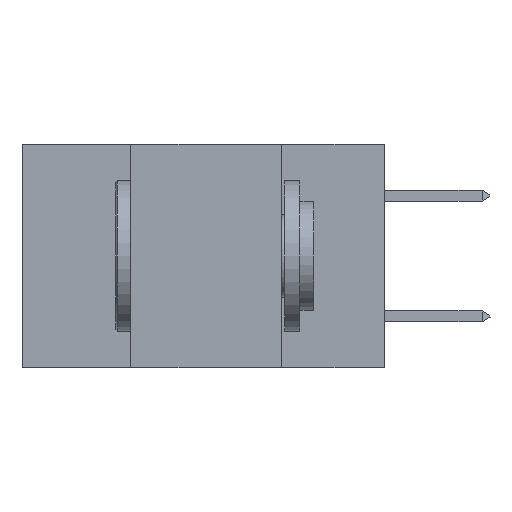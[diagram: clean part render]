
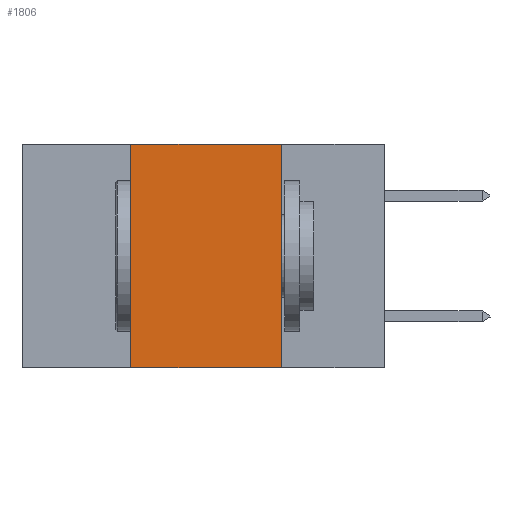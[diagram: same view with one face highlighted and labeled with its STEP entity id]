
A CAD part, left-side view. The second image highlights one B-rep face of the part: STEP entity #1806.
In plain terms, the highlighted planar face has unit normal (-1, 0, 0).
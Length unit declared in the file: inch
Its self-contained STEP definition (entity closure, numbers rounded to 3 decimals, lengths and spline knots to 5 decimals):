
#465 = CARTESIAN_POINT ( 'NONE',  ( 0., 0.42, 0. ) ) ;
#1806 = ADVANCED_FACE ( 'NONE', ( #6356 ), #15922, .F. ) ;
#1963 = ORIENTED_EDGE ( 'NONE', *, *, #30874, .F. ) ;
#4531 = CARTESIAN_POINT ( 'NONE',  ( 0., 0.17, -0.37 ) ) ;
#5035 = VECTOR ( 'NONE', #5827, 39.37008 ) ;
#5827 = DIRECTION ( 'NONE',  ( 0., 0., -1. ) ) ;
#6119 = LINE ( 'NONE', #32080, #33643 ) ;
#6356 = FACE_OUTER_BOUND ( 'NONE', #23006, .T. ) ;
#6683 = CARTESIAN_POINT ( 'NONE',  ( 0., 0.6, -0.37 ) ) ;
#7139 = DIRECTION ( 'NONE',  ( 0., 0., -1. ) ) ;
#7797 = VERTEX_POINT ( 'NONE', #34424 ) ;
#9125 = CARTESIAN_POINT ( 'NONE',  ( 0., 0.17, 0. ) ) ;
#10080 = VECTOR ( 'NONE', #25362, 39.37008 ) ;
#10627 = VERTEX_POINT ( 'NONE', #4531 ) ;
#11083 = CARTESIAN_POINT ( 'NONE',  ( 0., 0.6, 0. ) ) ;
#11844 = VECTOR ( 'NONE', #26947, 39.37008 ) ;
#12594 = VERTEX_POINT ( 'NONE', #9125 ) ;
#13259 = VERTEX_POINT ( 'NONE', #465 ) ;
#14514 = DIRECTION ( 'NONE',  ( 1., 0., 0. ) ) ;
#14752 = LINE ( 'NONE', #11083, #11844 ) ;
#15922 = PLANE ( 'NONE',  #28023 ) ;
#16336 = LINE ( 'NONE', #16603, #5035 ) ;
#16603 = CARTESIAN_POINT ( 'NONE',  ( 0., 0.17, 0. ) ) ;
#17176 = LINE ( 'NONE', #6683, #10080 ) ;
#18801 = DIRECTION ( 'NONE',  ( 0., 0., 1. ) ) ;
#23006 = EDGE_LOOP ( 'NONE', ( #31214, #28139, #1963, #32334 ) ) ;
#25010 = EDGE_CURVE ( 'NONE', #13259, #12594, #14752, .T. ) ;
#25362 = DIRECTION ( 'NONE',  ( 0., -1., 0. ) ) ;
#26947 = DIRECTION ( 'NONE',  ( 0., -1., 0. ) ) ;
#28023 = AXIS2_PLACEMENT_3D ( 'NONE', #33562, #14514, #7139 ) ;
#28139 = ORIENTED_EDGE ( 'NONE', *, *, #25010, .F. ) ;
#28446 = EDGE_CURVE ( 'NONE', #7797, #10627, #17176, .T. ) ;
#28940 = EDGE_CURVE ( 'NONE', #12594, #10627, #16336, .T. ) ;
#30874 = EDGE_CURVE ( 'NONE', #7797, #13259, #6119, .T. ) ;
#31214 = ORIENTED_EDGE ( 'NONE', *, *, #28940, .F. ) ;
#32080 = CARTESIAN_POINT ( 'NONE',  ( 0., 0.42, 0. ) ) ;
#32334 = ORIENTED_EDGE ( 'NONE', *, *, #28446, .T. ) ;
#33562 = CARTESIAN_POINT ( 'NONE',  ( 0., 0.6, 0. ) ) ;
#33643 = VECTOR ( 'NONE', #18801, 39.37008 ) ;
#34424 = CARTESIAN_POINT ( 'NONE',  ( 0., 0.42, -0.37 ) ) ;
